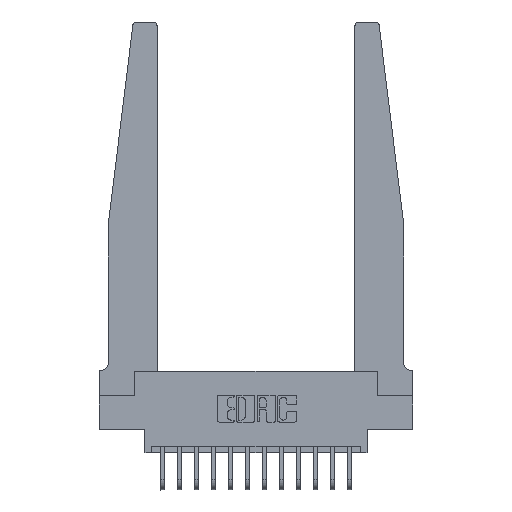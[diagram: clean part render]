
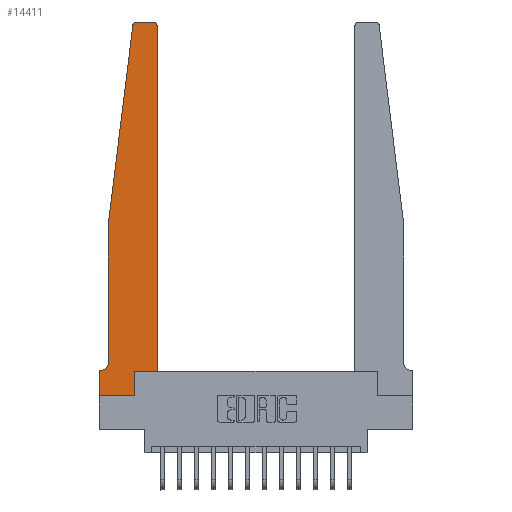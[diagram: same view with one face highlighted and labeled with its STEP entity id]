
A CAD part, top view. The second image highlights one B-rep face of the part: STEP entity #14411.
In plain terms, the highlighted planar face has unit normal (0, 0, 1).
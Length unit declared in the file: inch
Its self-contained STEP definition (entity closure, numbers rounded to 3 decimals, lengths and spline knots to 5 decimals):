
#210 = VECTOR ( 'NONE', #18187, 39.37008 ) ;
#238 = EDGE_LOOP ( 'NONE', ( #15950, #15997, #16060, #1049, #6518, #8102, #15396, #9469, #14102, #9538, #9013, #9932 ) ) ;
#326 = CARTESIAN_POINT ( 'NONE',  ( 0., 0.1875, 0.37 ) ) ;
#344 = EDGE_CURVE ( 'NONE', #6690, #5243, #3850, .T. ) ;
#637 = CARTESIAN_POINT ( 'NONE',  ( 0., 0., 0.37 ) ) ;
#1049 = ORIENTED_EDGE ( 'NONE', *, *, #3031, .T. ) ;
#1103 = FACE_OUTER_BOUND ( 'NONE', #238, .T. ) ;
#1409 = CARTESIAN_POINT ( 'NONE',  ( 0.015, 0.2375, 0.37 ) ) ;
#1454 = CARTESIAN_POINT ( 'NONE',  ( 0.27653, 2.75, 0.37 ) ) ;
#1495 = CARTESIAN_POINT ( 'NONE',  ( 0.2605, 0.18, 0.37 ) ) ;
#1670 = PLANE ( 'NONE',  #17602 ) ;
#1782 = DIRECTION ( 'NONE',  ( 0., 0., 1. ) ) ;
#1836 = DIRECTION ( 'NONE',  ( 1., 0., 0. ) ) ;
#1915 = EDGE_CURVE ( 'NONE', #13252, #12307, #18377, .T. ) ;
#1970 = CARTESIAN_POINT ( 'NONE',  ( 0.25, 2.75, 0.37 ) ) ;
#2138 = VERTEX_POINT ( 'NONE', #326 ) ;
#2227 = LINE ( 'NONE', #637, #15885 ) ;
#2882 = VECTOR ( 'NONE', #11667, 39.37008 ) ;
#2980 = DIRECTION ( 'NONE',  ( 0., 0., -1. ) ) ;
#3031 = EDGE_CURVE ( 'NONE', #15107, #6690, #9149, .T. ) ;
#3052 = AXIS2_PLACEMENT_3D ( 'NONE', #13376, #1782, #1836 ) ;
#3330 = DIRECTION ( 'NONE',  ( 0., -1., 0. ) ) ;
#3733 = CIRCLE ( 'NONE', #3052, 0.03 ) ;
#3819 = EDGE_CURVE ( 'NONE', #3894, #7088, #12486, .T. ) ;
#3850 = CIRCLE ( 'NONE', #15352, 0.05 ) ;
#3894 = VERTEX_POINT ( 'NONE', #4971 ) ;
#3909 = CARTESIAN_POINT ( 'NONE',  ( 0.065, 0.2375, 0.37 ) ) ;
#3925 = VERTEX_POINT ( 'NONE', #1495 ) ;
#3977 = VERTEX_POINT ( 'NONE', #5362 ) ;
#4362 = CARTESIAN_POINT ( 'NONE',  ( 0.065, 1.25, 0.37 ) ) ;
#4540 = CARTESIAN_POINT ( 'NONE',  ( 0., 0.1875, 0.37 ) ) ;
#4588 = CARTESIAN_POINT ( 'NONE',  ( 0.425, 0.18, 0.37 ) ) ;
#4902 = DIRECTION ( 'NONE',  ( -1., 0., 0. ) ) ;
#4971 = CARTESIAN_POINT ( 'NONE',  ( 0.395, 2.75, 0.37 ) ) ;
#5113 = LINE ( 'NONE', #6471, #14107 ) ;
#5243 = VERTEX_POINT ( 'NONE', #11018 ) ;
#5317 = DIRECTION ( 'NONE',  ( 0., -1., 0. ) ) ;
#5362 = CARTESIAN_POINT ( 'NONE',  ( 0.24675, 2.72367, 0.37 ) ) ;
#5599 = LINE ( 'NONE', #16726, #6947 ) ;
#5822 = CARTESIAN_POINT ( 'NONE',  ( 0., 0., 0.37 ) ) ;
#6471 = CARTESIAN_POINT ( 'NONE',  ( 0., 0., 0.37 ) ) ;
#6518 = ORIENTED_EDGE ( 'NONE', *, *, #344, .T. ) ;
#6690 = VERTEX_POINT ( 'NONE', #3909 ) ;
#6738 = LINE ( 'NONE', #9507, #13485 ) ;
#6926 = LINE ( 'NONE', #4362, #2882 ) ;
#6947 = VECTOR ( 'NONE', #8051, 39.37008 ) ;
#7088 = VERTEX_POINT ( 'NONE', #1454 ) ;
#7274 = CARTESIAN_POINT ( 'NONE',  ( 0.2605, 0., 0.37 ) ) ;
#7308 = DIRECTION ( 'NONE',  ( -1., 0., 0. ) ) ;
#7519 = EDGE_CURVE ( 'NONE', #3925, #13252, #14207, .T. ) ;
#8051 = DIRECTION ( 'NONE',  ( 0., 1., 0. ) ) ;
#8102 = ORIENTED_EDGE ( 'NONE', *, *, #9006, .T. ) ;
#8187 = CARTESIAN_POINT ( 'NONE',  ( 0.425, 0.18, 0.37 ) ) ;
#8214 = DIRECTION ( 'NONE',  ( -1., 0., 0. ) ) ;
#9006 = EDGE_CURVE ( 'NONE', #5243, #2138, #6738, .T. ) ;
#9013 = ORIENTED_EDGE ( 'NONE', *, *, #1915, .T. ) ;
#9149 = LINE ( 'NONE', #13628, #11372 ) ;
#9175 = CARTESIAN_POINT ( 'NONE',  ( 0.425, 0.18, 0.37 ) ) ;
#9469 = ORIENTED_EDGE ( 'NONE', *, *, #15322, .T. ) ;
#9507 = CARTESIAN_POINT ( 'NONE',  ( 0.065, 0.1875, 0.37 ) ) ;
#9538 = ORIENTED_EDGE ( 'NONE', *, *, #7519, .T. ) ;
#9558 = DIRECTION ( 'NONE',  ( 0., 0., 1. ) ) ;
#9754 = AXIS2_PLACEMENT_3D ( 'NONE', #14623, #9558, #11111 ) ;
#9837 = VERTEX_POINT ( 'NONE', #5822 ) ;
#9932 = ORIENTED_EDGE ( 'NONE', *, *, #10081, .T. ) ;
#10081 = EDGE_CURVE ( 'NONE', #12307, #3894, #3733, .T. ) ;
#10155 = DIRECTION ( 'NONE',  ( 0., 0., 1. ) ) ;
#10358 = CARTESIAN_POINT ( 'NONE',  ( 0.425, 2.72, 0.37 ) ) ;
#10490 = EDGE_CURVE ( 'NONE', #7088, #3977, #13835, .T. ) ;
#11018 = CARTESIAN_POINT ( 'NONE',  ( 0.015, 0.1875, 0.37 ) ) ;
#11111 = DIRECTION ( 'NONE',  ( 1., 0., 0. ) ) ;
#11372 = VECTOR ( 'NONE', #3330, 39.37008 ) ;
#11667 = DIRECTION ( 'NONE',  ( -0.122, -0.992, 0. ) ) ;
#11791 = VERTEX_POINT ( 'NONE', #7274 ) ;
#12307 = VERTEX_POINT ( 'NONE', #10358 ) ;
#12412 = DIRECTION ( 'NONE',  ( 1., 0., 0. ) ) ;
#12486 = LINE ( 'NONE', #1970, #16744 ) ;
#13252 = VERTEX_POINT ( 'NONE', #4588 ) ;
#13376 = CARTESIAN_POINT ( 'NONE',  ( 0.395, 2.72, 0.37 ) ) ;
#13485 = VECTOR ( 'NONE', #8214, 39.37008 ) ;
#13628 = CARTESIAN_POINT ( 'NONE',  ( 0.065, 1.25, 0.37 ) ) ;
#13835 = CIRCLE ( 'NONE', #9754, 0.03 ) ;
#14102 = ORIENTED_EDGE ( 'NONE', *, *, #17112, .T. ) ;
#14107 = VECTOR ( 'NONE', #12412, 39.37008 ) ;
#14207 = LINE ( 'NONE', #9175, #14651 ) ;
#14411 = ADVANCED_FACE ( 'NONE', ( #1103 ), #1670, .T. ) ;
#14623 = CARTESIAN_POINT ( 'NONE',  ( 0.27653, 2.72, 0.37 ) ) ;
#14651 = VECTOR ( 'NONE', #15037, 39.37008 ) ;
#14834 = EDGE_CURVE ( 'NONE', #3977, #15107, #6926, .T. ) ;
#15037 = DIRECTION ( 'NONE',  ( 1., 0., 0. ) ) ;
#15107 = VERTEX_POINT ( 'NONE', #16854 ) ;
#15322 = EDGE_CURVE ( 'NONE', #9837, #11791, #5113, .T. ) ;
#15352 = AXIS2_PLACEMENT_3D ( 'NONE', #1409, #2980, #7308 ) ;
#15396 = ORIENTED_EDGE ( 'NONE', *, *, #17578, .T. ) ;
#15885 = VECTOR ( 'NONE', #5317, 39.37008 ) ;
#15950 = ORIENTED_EDGE ( 'NONE', *, *, #3819, .T. ) ;
#15997 = ORIENTED_EDGE ( 'NONE', *, *, #10490, .T. ) ;
#16060 = ORIENTED_EDGE ( 'NONE', *, *, #14834, .T. ) ;
#16169 = DIRECTION ( 'NONE',  ( 1., 0., 0. ) ) ;
#16726 = CARTESIAN_POINT ( 'NONE',  ( 0.2605, 0.18, 0.37 ) ) ;
#16744 = VECTOR ( 'NONE', #4902, 39.37008 ) ;
#16854 = CARTESIAN_POINT ( 'NONE',  ( 0.065, 1.25, 0.37 ) ) ;
#17112 = EDGE_CURVE ( 'NONE', #11791, #3925, #5599, .T. ) ;
#17578 = EDGE_CURVE ( 'NONE', #2138, #9837, #2227, .T. ) ;
#17602 = AXIS2_PLACEMENT_3D ( 'NONE', #4540, #10155, #16169 ) ;
#18187 = DIRECTION ( 'NONE',  ( 0., 1., 0. ) ) ;
#18377 = LINE ( 'NONE', #8187, #210 ) ;
